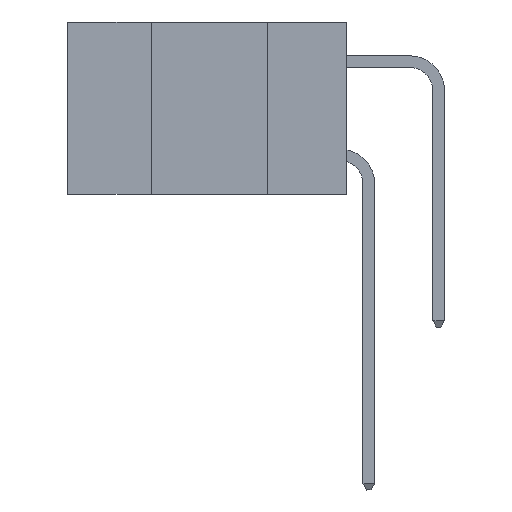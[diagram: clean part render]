
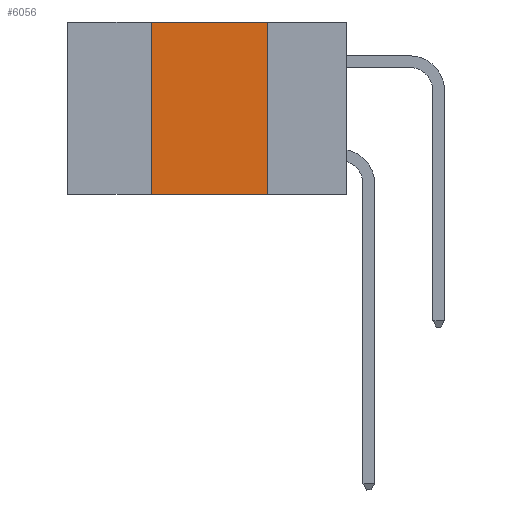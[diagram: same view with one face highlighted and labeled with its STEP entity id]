
A CAD part, left-side view. The second image highlights one B-rep face of the part: STEP entity #6056.
In plain terms, the highlighted planar face has unit normal (-1, 0, 0).
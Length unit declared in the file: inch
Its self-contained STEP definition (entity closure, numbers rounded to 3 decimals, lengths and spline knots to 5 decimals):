
#368 = ORIENTED_EDGE ( 'NONE', *, *, #3100, .F. ) ;
#375 = CARTESIAN_POINT ( 'NONE',  ( 0., 0.6, 0. ) ) ;
#719 = DIRECTION ( 'NONE',  ( 0., -1., 0. ) ) ;
#893 = EDGE_CURVE ( 'NONE', #3883, #8731, #6804, .T. ) ;
#1143 = VECTOR ( 'NONE', #719, 39.37008 ) ;
#1884 = VECTOR ( 'NONE', #10201, 39.37008 ) ;
#2341 = LINE ( 'NONE', #11005, #1143 ) ;
#2378 = PLANE ( 'NONE',  #3631 ) ;
#3100 = EDGE_CURVE ( 'NONE', #8731, #8617, #2341, .T. ) ;
#3159 = EDGE_CURVE ( 'NONE', #3883, #7245, #5875, .T. ) ;
#3162 = ORIENTED_EDGE ( 'NONE', *, *, #6811, .F. ) ;
#3335 = CARTESIAN_POINT ( 'NONE',  ( 0., 0.42, 0. ) ) ;
#3631 = AXIS2_PLACEMENT_3D ( 'NONE', #375, #7304, #4879 ) ;
#3883 = VERTEX_POINT ( 'NONE', #11109 ) ;
#4170 = CARTESIAN_POINT ( 'NONE',  ( 0., 0.42, 0. ) ) ;
#4879 = DIRECTION ( 'NONE',  ( 0., 0., -1. ) ) ;
#5375 = ORIENTED_EDGE ( 'NONE', *, *, #3159, .T. ) ;
#5875 = LINE ( 'NONE', #13267, #14202 ) ;
#6056 = ADVANCED_FACE ( 'NONE', ( #13274 ), #2378, .F. ) ;
#6229 = DIRECTION ( 'NONE',  ( 0., 0., -1. ) ) ;
#6358 = LINE ( 'NONE', #7356, #6541 ) ;
#6541 = VECTOR ( 'NONE', #6229, 39.37008 ) ;
#6804 = LINE ( 'NONE', #3335, #1884 ) ;
#6811 = EDGE_CURVE ( 'NONE', #8617, #7245, #6358, .T. ) ;
#7245 = VERTEX_POINT ( 'NONE', #9425 ) ;
#7304 = DIRECTION ( 'NONE',  ( 1., 0., 0. ) ) ;
#7356 = CARTESIAN_POINT ( 'NONE',  ( 0., 0.17, 0. ) ) ;
#7693 = DIRECTION ( 'NONE',  ( 0., -1., 0. ) ) ;
#8554 = EDGE_LOOP ( 'NONE', ( #3162, #368, #13699, #5375 ) ) ;
#8617 = VERTEX_POINT ( 'NONE', #12075 ) ;
#8731 = VERTEX_POINT ( 'NONE', #4170 ) ;
#9425 = CARTESIAN_POINT ( 'NONE',  ( 0., 0.17, -0.37 ) ) ;
#10201 = DIRECTION ( 'NONE',  ( 0., 0., 1. ) ) ;
#11005 = CARTESIAN_POINT ( 'NONE',  ( 0., 0.6, 0. ) ) ;
#11109 = CARTESIAN_POINT ( 'NONE',  ( 0., 0.42, -0.37 ) ) ;
#12075 = CARTESIAN_POINT ( 'NONE',  ( 0., 0.17, 0. ) ) ;
#13267 = CARTESIAN_POINT ( 'NONE',  ( 0., 0.6, -0.37 ) ) ;
#13274 = FACE_OUTER_BOUND ( 'NONE', #8554, .T. ) ;
#13699 = ORIENTED_EDGE ( 'NONE', *, *, #893, .F. ) ;
#14202 = VECTOR ( 'NONE', #7693, 39.37008 ) ;
